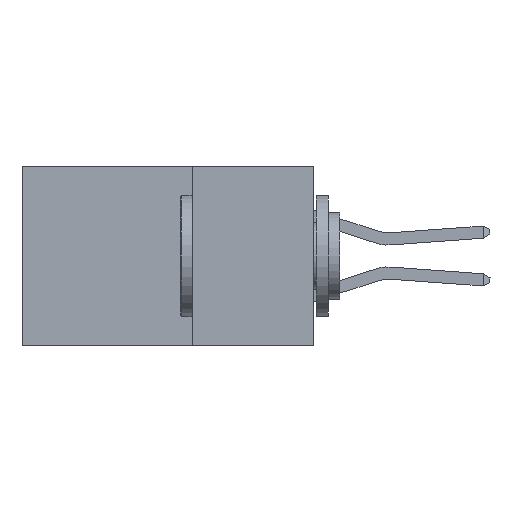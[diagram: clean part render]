
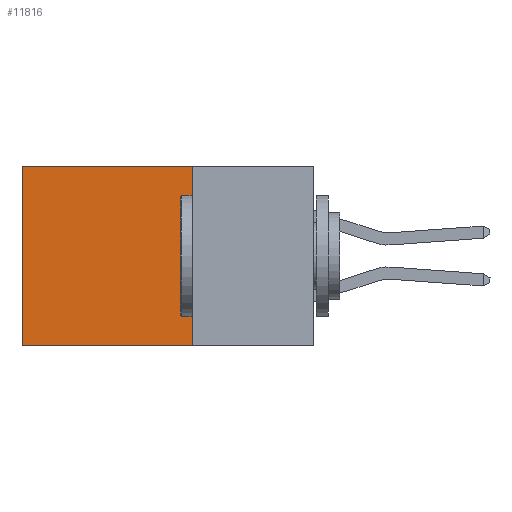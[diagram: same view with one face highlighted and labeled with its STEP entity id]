
A CAD part, left-side view. The second image highlights one B-rep face of the part: STEP entity #11816.
In plain terms, the highlighted planar face has unit normal (-1, 0, 0).
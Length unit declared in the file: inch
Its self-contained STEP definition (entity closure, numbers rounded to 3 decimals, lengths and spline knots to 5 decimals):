
#394 = EDGE_LOOP ( 'NONE', ( #1728, #499, #12849, #12191 ) ) ;
#499 = ORIENTED_EDGE ( 'NONE', *, *, #11203, .F. ) ;
#530 = EDGE_CURVE ( 'NONE', #9740, #4029, #6661, .T. ) ;
#654 = PLANE ( 'NONE',  #10919 ) ;
#1009 = LINE ( 'NONE', #3889, #6783 ) ;
#1062 = CARTESIAN_POINT ( 'NONE',  ( 0.2875, 0.25, -0.37 ) ) ;
#1452 = VECTOR ( 'NONE', #3977, 39.37008 ) ;
#1462 = CARTESIAN_POINT ( 'NONE',  ( 0.2875, 0.6, -0.37 ) ) ;
#1508 = CARTESIAN_POINT ( 'NONE',  ( 0.2875, 0.25, -0.37 ) ) ;
#1728 = ORIENTED_EDGE ( 'NONE', *, *, #10166, .T. ) ;
#2124 = EDGE_CURVE ( 'NONE', #9740, #10132, #2850, .T. ) ;
#2711 = FACE_OUTER_BOUND ( 'NONE', #394, .T. ) ;
#2850 = LINE ( 'NONE', #5232, #4855 ) ;
#3461 = CARTESIAN_POINT ( 'NONE',  ( 0.2875, 0.25, 0. ) ) ;
#3889 = CARTESIAN_POINT ( 'NONE',  ( 0.2875, 0.6, 0. ) ) ;
#3970 = DIRECTION ( 'NONE',  ( 0., 0., -1. ) ) ;
#3977 = DIRECTION ( 'NONE',  ( 0., 1., 0. ) ) ;
#4029 = VERTEX_POINT ( 'NONE', #1508 ) ;
#4670 = DIRECTION ( 'NONE',  ( 0., 0., -1. ) ) ;
#4855 = VECTOR ( 'NONE', #10153, 39.37008 ) ;
#5232 = CARTESIAN_POINT ( 'NONE',  ( 0.2875, 0.25, 0. ) ) ;
#5662 = DIRECTION ( 'NONE',  ( 1., 0., 0. ) ) ;
#5756 = VERTEX_POINT ( 'NONE', #1462 ) ;
#6442 = LINE ( 'NONE', #1062, #1452 ) ;
#6661 = LINE ( 'NONE', #10721, #10079 ) ;
#6783 = VECTOR ( 'NONE', #3970, 39.37008 ) ;
#7540 = DIRECTION ( 'NONE',  ( 0., 0., -1. ) ) ;
#7991 = CARTESIAN_POINT ( 'NONE',  ( 0.2875, 0.6, 0. ) ) ;
#9740 = VERTEX_POINT ( 'NONE', #3461 ) ;
#10079 = VECTOR ( 'NONE', #4670, 39.37008 ) ;
#10132 = VERTEX_POINT ( 'NONE', #7991 ) ;
#10153 = DIRECTION ( 'NONE',  ( 0., 1., 0. ) ) ;
#10166 = EDGE_CURVE ( 'NONE', #10132, #5756, #1009, .T. ) ;
#10721 = CARTESIAN_POINT ( 'NONE',  ( 0.2875, 0.25, 0. ) ) ;
#10919 = AXIS2_PLACEMENT_3D ( 'NONE', #11633, #5662, #7540 ) ;
#11203 = EDGE_CURVE ( 'NONE', #4029, #5756, #6442, .T. ) ;
#11633 = CARTESIAN_POINT ( 'NONE',  ( 0.2875, 0.25, 0. ) ) ;
#11816 = ADVANCED_FACE ( 'NONE', ( #2711 ), #654, .F. ) ;
#12191 = ORIENTED_EDGE ( 'NONE', *, *, #2124, .T. ) ;
#12849 = ORIENTED_EDGE ( 'NONE', *, *, #530, .F. ) ;
